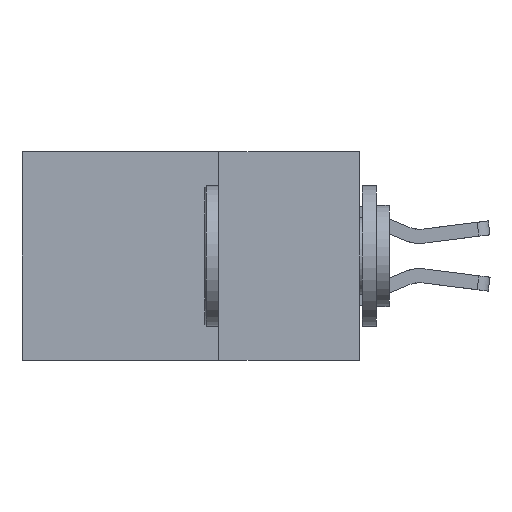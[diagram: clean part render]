
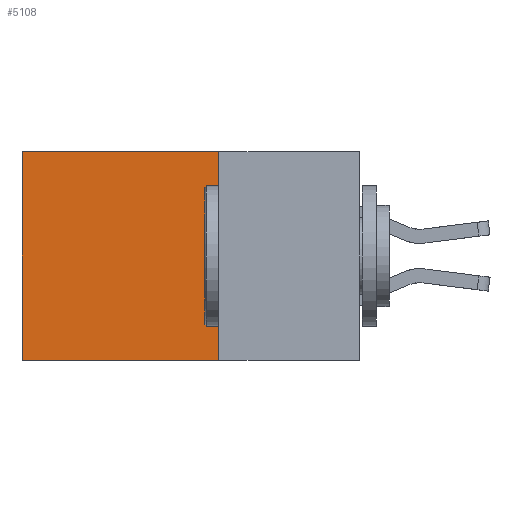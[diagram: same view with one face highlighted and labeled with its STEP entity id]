
A CAD part, left-side view. The second image highlights one B-rep face of the part: STEP entity #5108.
In plain terms, the highlighted planar face has unit normal (-1, 0, 0).
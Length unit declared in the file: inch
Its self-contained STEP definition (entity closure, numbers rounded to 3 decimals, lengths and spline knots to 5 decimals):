
#334 = VERTEX_POINT ( 'NONE', #11742 ) ;
#594 = CARTESIAN_POINT ( 'NONE',  ( 0.2875, 0.6, 0. ) ) ;
#1062 = CARTESIAN_POINT ( 'NONE',  ( 0.2875, 0.25, 0. ) ) ;
#1074 = ORIENTED_EDGE ( 'NONE', *, *, #3661, .T. ) ;
#1449 = DIRECTION ( 'NONE',  ( 0., 1., 0. ) ) ;
#1521 = DIRECTION ( 'NONE',  ( 1., 0., 0. ) ) ;
#1556 = DIRECTION ( 'NONE',  ( 0., 0., -1. ) ) ;
#1613 = FACE_OUTER_BOUND ( 'NONE', #4698, .T. ) ;
#2730 = DIRECTION ( 'NONE',  ( 0., 0., -1. ) ) ;
#2895 = PLANE ( 'NONE',  #4749 ) ;
#3351 = LINE ( 'NONE', #7692, #5067 ) ;
#3527 = LINE ( 'NONE', #594, #5380 ) ;
#3661 = EDGE_CURVE ( 'NONE', #8733, #334, #3851, .T. ) ;
#3694 = ORIENTED_EDGE ( 'NONE', *, *, #5050, .F. ) ;
#3745 = VERTEX_POINT ( 'NONE', #9648 ) ;
#3851 = LINE ( 'NONE', #6258, #8203 ) ;
#4698 = EDGE_LOOP ( 'NONE', ( #5828, #7349, #3694, #1074 ) ) ;
#4749 = AXIS2_PLACEMENT_3D ( 'NONE', #11153, #1521, #1556 ) ;
#5050 = EDGE_CURVE ( 'NONE', #8733, #3745, #5370, .T. ) ;
#5067 = VECTOR ( 'NONE', #1449, 39.37008 ) ;
#5081 = VECTOR ( 'NONE', #2730, 39.37008 ) ;
#5108 = ADVANCED_FACE ( 'NONE', ( #1613 ), #2895, .F. ) ;
#5370 = LINE ( 'NONE', #6452, #5081 ) ;
#5380 = VECTOR ( 'NONE', #7076, 39.37008 ) ;
#5528 = VERTEX_POINT ( 'NONE', #8757 ) ;
#5772 = EDGE_CURVE ( 'NONE', #3745, #5528, #3351, .T. ) ;
#5828 = ORIENTED_EDGE ( 'NONE', *, *, #10387, .T. ) ;
#6258 = CARTESIAN_POINT ( 'NONE',  ( 0.2875, 0.25, 0. ) ) ;
#6452 = CARTESIAN_POINT ( 'NONE',  ( 0.2875, 0.25, 0. ) ) ;
#7076 = DIRECTION ( 'NONE',  ( 0., 0., -1. ) ) ;
#7349 = ORIENTED_EDGE ( 'NONE', *, *, #5772, .F. ) ;
#7692 = CARTESIAN_POINT ( 'NONE',  ( 0.2875, 0.25, -0.37 ) ) ;
#8203 = VECTOR ( 'NONE', #11740, 39.37008 ) ;
#8733 = VERTEX_POINT ( 'NONE', #1062 ) ;
#8757 = CARTESIAN_POINT ( 'NONE',  ( 0.2875, 0.6, -0.37 ) ) ;
#9648 = CARTESIAN_POINT ( 'NONE',  ( 0.2875, 0.25, -0.37 ) ) ;
#10387 = EDGE_CURVE ( 'NONE', #334, #5528, #3527, .T. ) ;
#11153 = CARTESIAN_POINT ( 'NONE',  ( 0.2875, 0.25, 0. ) ) ;
#11740 = DIRECTION ( 'NONE',  ( 0., 1., 0. ) ) ;
#11742 = CARTESIAN_POINT ( 'NONE',  ( 0.2875, 0.6, 0. ) ) ;
